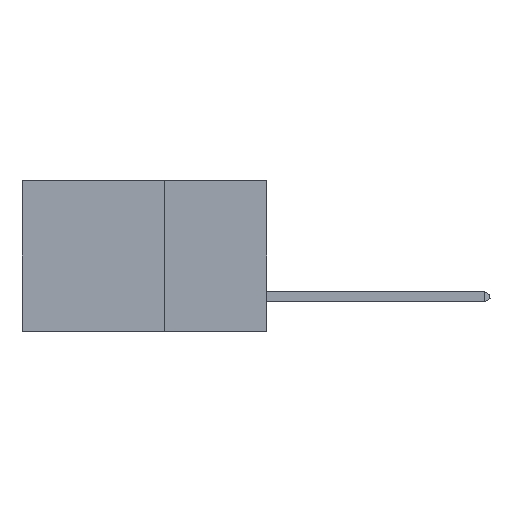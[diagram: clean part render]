
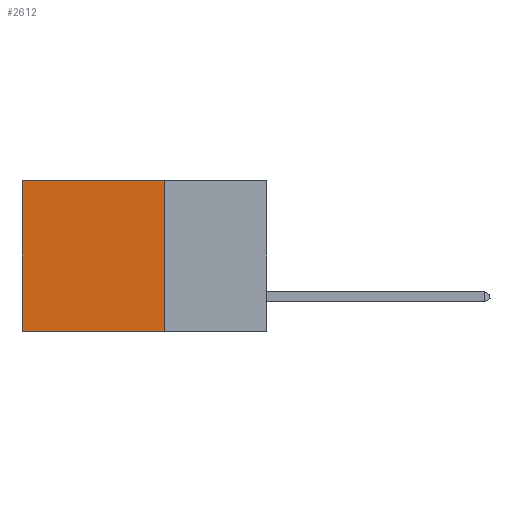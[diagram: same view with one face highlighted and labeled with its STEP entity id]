
A CAD part, left-side view. The second image highlights one B-rep face of the part: STEP entity #2612.
In plain terms, the highlighted planar face has unit normal (-1, 0, 0).
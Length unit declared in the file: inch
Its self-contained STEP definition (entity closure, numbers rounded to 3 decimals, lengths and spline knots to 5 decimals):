
#92 = LINE ( 'NONE', #28489, #27770 ) ;
#700 = VERTEX_POINT ( 'NONE', #23176 ) ;
#1022 = CARTESIAN_POINT ( 'NONE',  ( 0.2875, 0.6, 0. ) ) ;
#1096 = VERTEX_POINT ( 'NONE', #27402 ) ;
#2127 = DIRECTION ( 'NONE',  ( 1., 0., 0. ) ) ;
#2304 = LINE ( 'NONE', #31427, #22027 ) ;
#2612 = ADVANCED_FACE ( 'NONE', ( #10507 ), #26390, .F. ) ;
#3176 = EDGE_CURVE ( 'NONE', #12207, #25411, #25579, .T. ) ;
#10507 = FACE_OUTER_BOUND ( 'NONE', #27235, .T. ) ;
#10976 = VECTOR ( 'NONE', #14333, 39.37008 ) ;
#12172 = DIRECTION ( 'NONE',  ( 0., 1., 0. ) ) ;
#12207 = VERTEX_POINT ( 'NONE', #27606 ) ;
#13529 = LINE ( 'NONE', #1022, #10976 ) ;
#13886 = ORIENTED_EDGE ( 'NONE', *, *, #15631, .T. ) ;
#14333 = DIRECTION ( 'NONE',  ( 0., 0., -1. ) ) ;
#15352 = EDGE_CURVE ( 'NONE', #12207, #1096, #92, .T. ) ;
#15631 = EDGE_CURVE ( 'NONE', #25411, #700, #13529, .T. ) ;
#15664 = CARTESIAN_POINT ( 'NONE',  ( 0.2875, 0.25, 0. ) ) ;
#15704 = CARTESIAN_POINT ( 'NONE',  ( 0.2875, 0.25, 0. ) ) ;
#18114 = DIRECTION ( 'NONE',  ( 0., 0., -1. ) ) ;
#20841 = EDGE_CURVE ( 'NONE', #1096, #700, #2304, .T. ) ;
#21078 = CARTESIAN_POINT ( 'NONE',  ( 0.2875, 0.6, 0. ) ) ;
#21114 = DIRECTION ( 'NONE',  ( 0., 0., -1. ) ) ;
#22027 = VECTOR ( 'NONE', #12172, 39.37008 ) ;
#23176 = CARTESIAN_POINT ( 'NONE',  ( 0.2875, 0.6, -0.37 ) ) ;
#25154 = VECTOR ( 'NONE', #34500, 39.37008 ) ;
#25411 = VERTEX_POINT ( 'NONE', #21078 ) ;
#25579 = LINE ( 'NONE', #15704, #25154 ) ;
#26046 = ORIENTED_EDGE ( 'NONE', *, *, #20841, .F. ) ;
#26390 = PLANE ( 'NONE',  #26666 ) ;
#26666 = AXIS2_PLACEMENT_3D ( 'NONE', #15664, #2127, #21114 ) ;
#27235 = EDGE_LOOP ( 'NONE', ( #13886, #26046, #30071, #29739 ) ) ;
#27402 = CARTESIAN_POINT ( 'NONE',  ( 0.2875, 0.25, -0.37 ) ) ;
#27606 = CARTESIAN_POINT ( 'NONE',  ( 0.2875, 0.25, 0. ) ) ;
#27770 = VECTOR ( 'NONE', #18114, 39.37008 ) ;
#28489 = CARTESIAN_POINT ( 'NONE',  ( 0.2875, 0.25, 0. ) ) ;
#29739 = ORIENTED_EDGE ( 'NONE', *, *, #3176, .T. ) ;
#30071 = ORIENTED_EDGE ( 'NONE', *, *, #15352, .F. ) ;
#31427 = CARTESIAN_POINT ( 'NONE',  ( 0.2875, 0.25, -0.37 ) ) ;
#34500 = DIRECTION ( 'NONE',  ( 0., 1., 0. ) ) ;
